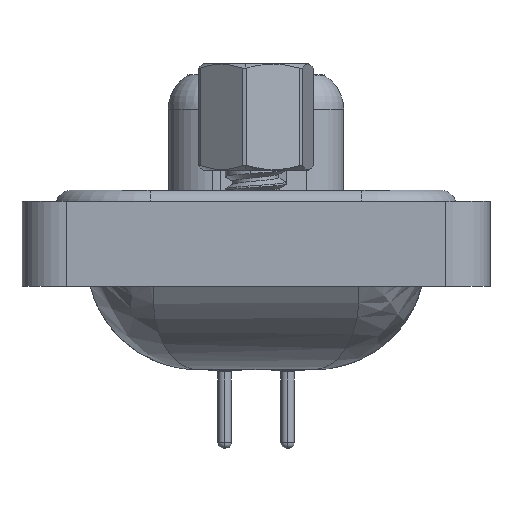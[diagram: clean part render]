
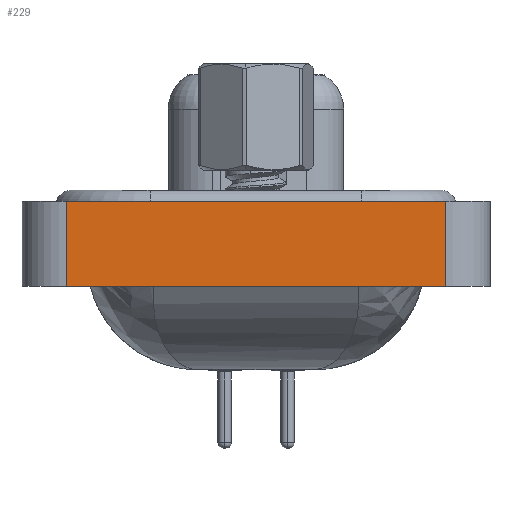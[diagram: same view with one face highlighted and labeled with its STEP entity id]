
A CAD part, left-side view. The second image highlights one B-rep face of the part: STEP entity #229.
In plain terms, the highlighted planar face has unit normal (-1, 0, 0).
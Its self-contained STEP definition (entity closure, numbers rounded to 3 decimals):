
#229 = ADVANCED_FACE ( 'NONE', ( #3063 ), #1255, .T. ) ;
#583 = ORIENTED_EDGE ( 'NONE', *, *, #6844, .T. ) ;
#1255 = PLANE ( 'NONE',  #1635 ) ;
#1635 = AXIS2_PLACEMENT_3D ( 'NONE', #23409, #10389, #8767 ) ;
#1773 = CARTESIAN_POINT ( 'NONE',  ( -7.35, -8.55, 0.5 ) ) ;
#2366 = EDGE_CURVE ( 'NONE', #11645, #14534, #20365, .T. ) ;
#2697 = VECTOR ( 'NONE', #17636, 1000. ) ;
#3063 = FACE_OUTER_BOUND ( 'NONE', #5563, .T. ) ;
#3627 = LINE ( 'NONE', #1773, #23991 ) ;
#5563 = EDGE_LOOP ( 'NONE', ( #22898, #15993, #17656, #583 ) ) ;
#5742 = CARTESIAN_POINT ( 'NONE',  ( -7.35, 8.55, 0.5 ) ) ;
#6490 = CARTESIAN_POINT ( 'NONE',  ( -7.35, 8.55, -3.35 ) ) ;
#6844 = EDGE_CURVE ( 'NONE', #23361, #11645, #21192, .T. ) ;
#7076 = DIRECTION ( 'NONE',  ( 0., -1., 0. ) ) ;
#8767 = DIRECTION ( 'NONE',  ( 0., 0., 1. ) ) ;
#10389 = DIRECTION ( 'NONE',  ( -1., 0., 0. ) ) ;
#11183 = EDGE_CURVE ( 'NONE', #23361, #23555, #17479, .T. ) ;
#11645 = VERTEX_POINT ( 'NONE', #21107 ) ;
#12010 = CARTESIAN_POINT ( 'NONE',  ( -7.35, -8.55, -3.35 ) ) ;
#13230 = EDGE_CURVE ( 'NONE', #23555, #14534, #3627, .T. ) ;
#14534 = VERTEX_POINT ( 'NONE', #19686 ) ;
#14852 = CARTESIAN_POINT ( 'NONE',  ( -7.35, -8.55, -3.35 ) ) ;
#15993 = ORIENTED_EDGE ( 'NONE', *, *, #13230, .F. ) ;
#17479 = LINE ( 'NONE', #6490, #21798 ) ;
#17636 = DIRECTION ( 'NONE',  ( 0., -1., 0. ) ) ;
#17656 = ORIENTED_EDGE ( 'NONE', *, *, #11183, .F. ) ;
#17832 = DIRECTION ( 'NONE',  ( 0., 0., 1. ) ) ;
#18390 = DIRECTION ( 'NONE',  ( 0., 0., 1. ) ) ;
#19686 = CARTESIAN_POINT ( 'NONE',  ( -7.35, -8.55, 0.5 ) ) ;
#20365 = LINE ( 'NONE', #14852, #22488 ) ;
#21107 = CARTESIAN_POINT ( 'NONE',  ( -7.35, -8.55, -3.35 ) ) ;
#21192 = LINE ( 'NONE', #12010, #2697 ) ;
#21798 = VECTOR ( 'NONE', #17832, 1000. ) ;
#22153 = CARTESIAN_POINT ( 'NONE',  ( -7.35, 8.55, -3.35 ) ) ;
#22488 = VECTOR ( 'NONE', #18390, 1000. ) ;
#22898 = ORIENTED_EDGE ( 'NONE', *, *, #2366, .T. ) ;
#23361 = VERTEX_POINT ( 'NONE', #22153 ) ;
#23409 = CARTESIAN_POINT ( 'NONE',  ( -7.35, -8.55, -3.35 ) ) ;
#23555 = VERTEX_POINT ( 'NONE', #5742 ) ;
#23991 = VECTOR ( 'NONE', #7076, 1000. ) ;
